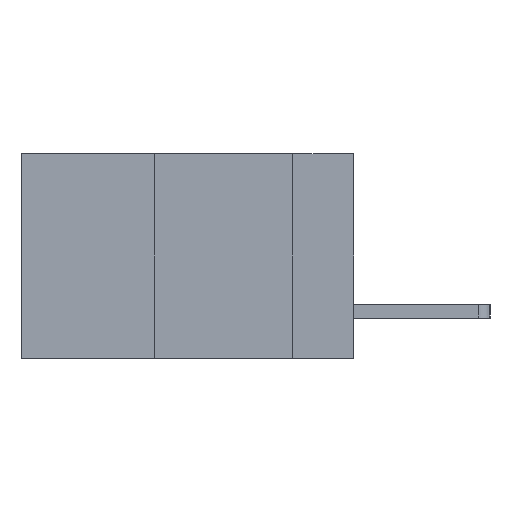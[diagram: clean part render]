
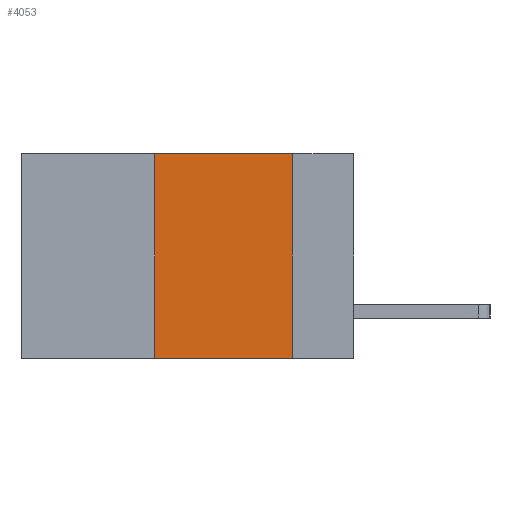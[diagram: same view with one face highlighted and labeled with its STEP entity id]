
A CAD part, left-side view. The second image highlights one B-rep face of the part: STEP entity #4053.
In plain terms, the highlighted planar face has unit normal (-1, 0, 0).
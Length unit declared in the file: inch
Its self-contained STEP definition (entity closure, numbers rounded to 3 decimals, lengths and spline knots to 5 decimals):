
#526 = CARTESIAN_POINT ( 'NONE',  ( 0., 0.6, 0. ) ) ;
#1931 = DIRECTION ( 'NONE',  ( 0., 0., -1. ) ) ;
#2174 = CARTESIAN_POINT ( 'NONE',  ( 0., 0.36, 0. ) ) ;
#2445 = VERTEX_POINT ( 'NONE', #7613 ) ;
#2668 = PLANE ( 'NONE',  #3994 ) ;
#2697 = CARTESIAN_POINT ( 'NONE',  ( 0., 0.36, 0. ) ) ;
#2939 = LINE ( 'NONE', #6073, #11762 ) ;
#3658 = VERTEX_POINT ( 'NONE', #2697 ) ;
#3994 = AXIS2_PLACEMENT_3D ( 'NONE', #10909, #4725, #8793 ) ;
#3998 = EDGE_CURVE ( 'NONE', #3658, #11780, #4787, .T. ) ;
#4053 = ADVANCED_FACE ( 'NONE', ( #9709 ), #2668, .F. ) ;
#4311 = DIRECTION ( 'NONE',  ( 0., 0., 1. ) ) ;
#4381 = ORIENTED_EDGE ( 'NONE', *, *, #10573, .F. ) ;
#4446 = LINE ( 'NONE', #2174, #6158 ) ;
#4725 = DIRECTION ( 'NONE',  ( 1., 0., 0. ) ) ;
#4787 = LINE ( 'NONE', #526, #9297 ) ;
#4942 = LINE ( 'NONE', #9004, #8542 ) ;
#5427 = EDGE_LOOP ( 'NONE', ( #4381, #8532, #6783, #9228 ) ) ;
#5915 = CARTESIAN_POINT ( 'NONE',  ( 0., 0.11, 0. ) ) ;
#5931 = EDGE_CURVE ( 'NONE', #7867, #3658, #4446, .T. ) ;
#6073 = CARTESIAN_POINT ( 'NONE',  ( 0., 0.11, 0. ) ) ;
#6158 = VECTOR ( 'NONE', #4311, 39.37008 ) ;
#6783 = ORIENTED_EDGE ( 'NONE', *, *, #5931, .F. ) ;
#7613 = CARTESIAN_POINT ( 'NONE',  ( 0., 0.11, -0.37 ) ) ;
#7867 = VERTEX_POINT ( 'NONE', #8821 ) ;
#8532 = ORIENTED_EDGE ( 'NONE', *, *, #3998, .F. ) ;
#8542 = VECTOR ( 'NONE', #10793, 39.37008 ) ;
#8591 = EDGE_CURVE ( 'NONE', #7867, #2445, #4942, .T. ) ;
#8793 = DIRECTION ( 'NONE',  ( 0., 0., -1. ) ) ;
#8821 = CARTESIAN_POINT ( 'NONE',  ( 0., 0.36, -0.37 ) ) ;
#8856 = DIRECTION ( 'NONE',  ( 0., -1., 0. ) ) ;
#9004 = CARTESIAN_POINT ( 'NONE',  ( 0., 0.6, -0.37 ) ) ;
#9228 = ORIENTED_EDGE ( 'NONE', *, *, #8591, .T. ) ;
#9297 = VECTOR ( 'NONE', #8856, 39.37008 ) ;
#9709 = FACE_OUTER_BOUND ( 'NONE', #5427, .T. ) ;
#10573 = EDGE_CURVE ( 'NONE', #11780, #2445, #2939, .T. ) ;
#10793 = DIRECTION ( 'NONE',  ( 0., -1., 0. ) ) ;
#10909 = CARTESIAN_POINT ( 'NONE',  ( 0., 0.6, 0. ) ) ;
#11762 = VECTOR ( 'NONE', #1931, 39.37008 ) ;
#11780 = VERTEX_POINT ( 'NONE', #5915 ) ;
